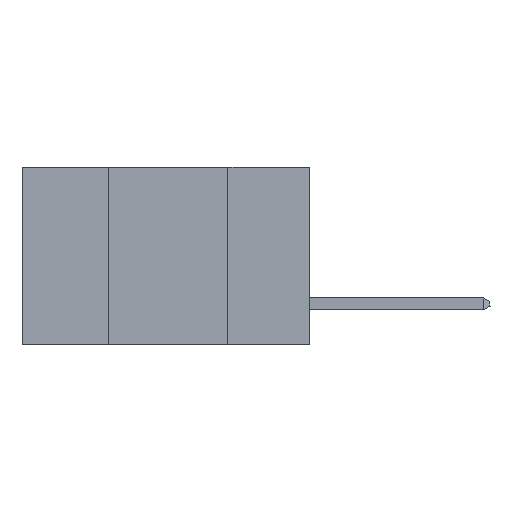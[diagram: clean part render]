
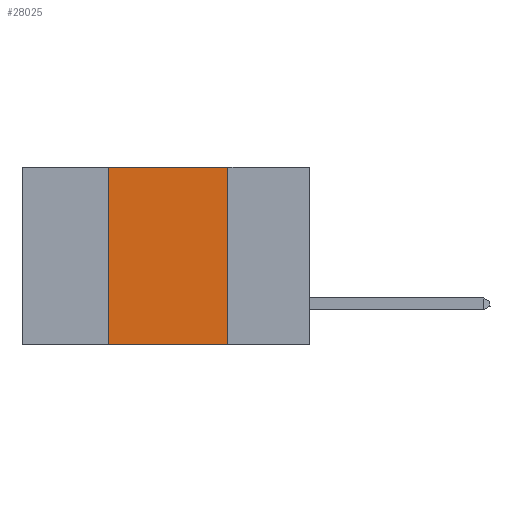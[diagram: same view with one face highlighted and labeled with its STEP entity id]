
A CAD part, left-side view. The second image highlights one B-rep face of the part: STEP entity #28025.
In plain terms, the highlighted planar face has unit normal (-1, 0, 0).
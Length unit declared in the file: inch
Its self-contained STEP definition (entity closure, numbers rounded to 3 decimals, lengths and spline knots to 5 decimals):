
#231 = PLANE ( 'NONE',  #19274 ) ;
#831 = CARTESIAN_POINT ( 'NONE',  ( 0., 0.17, 0. ) ) ;
#1457 = DIRECTION ( 'NONE',  ( 0., 0., -1. ) ) ;
#3860 = DIRECTION ( 'NONE',  ( 0., 0., -1. ) ) ;
#5010 = CARTESIAN_POINT ( 'NONE',  ( 0., 0.6, -0.37 ) ) ;
#5092 = EDGE_CURVE ( 'NONE', #24365, #46361, #22296, .T. ) ;
#5148 = FACE_OUTER_BOUND ( 'NONE', #36863, .T. ) ;
#6067 = VECTOR ( 'NONE', #20325, 39.37008 ) ;
#7180 = EDGE_CURVE ( 'NONE', #29639, #46361, #44279, .T. ) ;
#7393 = EDGE_CURVE ( 'NONE', #24365, #12562, #41969, .T. ) ;
#8448 = CARTESIAN_POINT ( 'NONE',  ( 0., 0.17, 0. ) ) ;
#12562 = VERTEX_POINT ( 'NONE', #34171 ) ;
#13736 = CARTESIAN_POINT ( 'NONE',  ( 0., 0.42, -0.37 ) ) ;
#14328 = ORIENTED_EDGE ( 'NONE', *, *, #7180, .F. ) ;
#17826 = CARTESIAN_POINT ( 'NONE',  ( 0., 0.17, -0.37 ) ) ;
#19274 = AXIS2_PLACEMENT_3D ( 'NONE', #33349, #29532, #3860 ) ;
#19691 = DIRECTION ( 'NONE',  ( 0., -1., 0. ) ) ;
#20325 = DIRECTION ( 'NONE',  ( 0., -1., 0. ) ) ;
#21550 = LINE ( 'NONE', #31317, #6067 ) ;
#22296 = LINE ( 'NONE', #5010, #31960 ) ;
#24365 = VERTEX_POINT ( 'NONE', #13736 ) ;
#25056 = ORIENTED_EDGE ( 'NONE', *, *, #5092, .T. ) ;
#25460 = DIRECTION ( 'NONE',  ( 0., 0., 1. ) ) ;
#28025 = ADVANCED_FACE ( 'NONE', ( #5148 ), #231, .F. ) ;
#29532 = DIRECTION ( 'NONE',  ( 1., 0., 0. ) ) ;
#29639 = VERTEX_POINT ( 'NONE', #8448 ) ;
#31317 = CARTESIAN_POINT ( 'NONE',  ( 0., 0.6, 0. ) ) ;
#31960 = VECTOR ( 'NONE', #19691, 39.37008 ) ;
#33349 = CARTESIAN_POINT ( 'NONE',  ( 0., 0.6, 0. ) ) ;
#34171 = CARTESIAN_POINT ( 'NONE',  ( 0., 0.42, 0. ) ) ;
#36311 = CARTESIAN_POINT ( 'NONE',  ( 0., 0.42, 0. ) ) ;
#36863 = EDGE_LOOP ( 'NONE', ( #14328, #40211, #38757, #25056 ) ) ;
#37005 = EDGE_CURVE ( 'NONE', #12562, #29639, #21550, .T. ) ;
#38757 = ORIENTED_EDGE ( 'NONE', *, *, #7393, .F. ) ;
#40211 = ORIENTED_EDGE ( 'NONE', *, *, #37005, .F. ) ;
#41445 = VECTOR ( 'NONE', #1457, 39.37008 ) ;
#41969 = LINE ( 'NONE', #36311, #44258 ) ;
#44258 = VECTOR ( 'NONE', #25460, 39.37008 ) ;
#44279 = LINE ( 'NONE', #831, #41445 ) ;
#46361 = VERTEX_POINT ( 'NONE', #17826 ) ;
